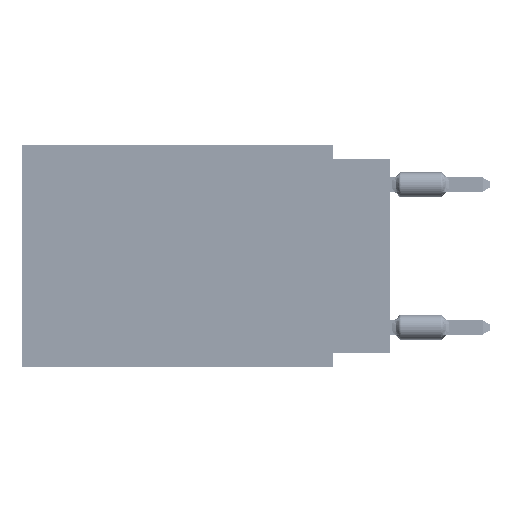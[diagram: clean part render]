
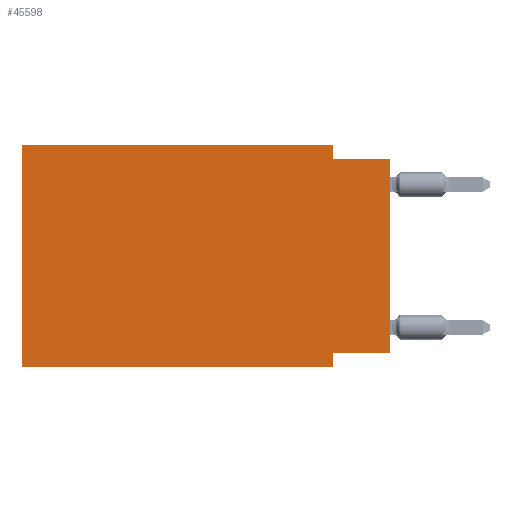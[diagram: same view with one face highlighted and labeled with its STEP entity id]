
A CAD part, left-side view. The second image highlights one B-rep face of the part: STEP entity #45598.
In plain terms, the highlighted planar face has unit normal (-1, 0, 0).
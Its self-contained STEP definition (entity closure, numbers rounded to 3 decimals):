
#2475 = DIRECTION ( 'NONE',  ( 0., -1., 0. ) ) ;
#2981 = EDGE_CURVE ( 'NONE', #34282, #34137, #37759, .T. ) ;
#3717 = VECTOR ( 'NONE', #36213, 1000. ) ;
#3864 = FACE_OUTER_BOUND ( 'NONE', #32649, .T. ) ;
#4817 = VECTOR ( 'NONE', #51112, 1000. ) ;
#5017 = DIRECTION ( 'NONE',  ( 0., -1., 0. ) ) ;
#6889 = EDGE_CURVE ( 'NONE', #23147, #39089, #38654, .T. ) ;
#7675 = VECTOR ( 'NONE', #46859, 1000. ) ;
#10499 = CARTESIAN_POINT ( 'NONE',  ( 0., 0., -0.635 ) ) ;
#12782 = CARTESIAN_POINT ( 'NONE',  ( 0., 0., -9.271 ) ) ;
#13232 = EDGE_CURVE ( 'NONE', #24584, #39089, #41303, .T. ) ;
#13261 = ORIENTED_EDGE ( 'NONE', *, *, #19563, .F. ) ;
#13818 = ORIENTED_EDGE ( 'NONE', *, *, #63103, .T. ) ;
#16431 = EDGE_CURVE ( 'NONE', #24584, #31698, #51775, .T. ) ;
#17230 = EDGE_CURVE ( 'NONE', #31698, #34282, #43219, .T. ) ;
#17714 = VECTOR ( 'NONE', #5017, 1000. ) ;
#19563 = EDGE_CURVE ( 'NONE', #34137, #33366, #47447, .T. ) ;
#22340 = CARTESIAN_POINT ( 'NONE',  ( 0., 2.54, 0. ) ) ;
#22979 = VECTOR ( 'NONE', #62501, 1000. ) ;
#23147 = VERTEX_POINT ( 'NONE', #27498 ) ;
#24584 = VERTEX_POINT ( 'NONE', #31241 ) ;
#26050 = DIRECTION ( 'NONE',  ( 0., 1., 0. ) ) ;
#27498 = CARTESIAN_POINT ( 'NONE',  ( 0., 2.54, -9.271 ) ) ;
#27573 = CARTESIAN_POINT ( 'NONE',  ( 0., 0., -0.635 ) ) ;
#27661 = VECTOR ( 'NONE', #2475, 1000. ) ;
#28936 = VECTOR ( 'NONE', #26050, 1000. ) ;
#30209 = PLANE ( 'NONE',  #43224 ) ;
#30893 = VECTOR ( 'NONE', #32599, 1000. ) ;
#31241 = CARTESIAN_POINT ( 'NONE',  ( 0., 16.383, -9.906 ) ) ;
#31698 = VERTEX_POINT ( 'NONE', #35308 ) ;
#32599 = DIRECTION ( 'NONE',  ( 0., 0., -1. ) ) ;
#32649 = EDGE_LOOP ( 'NONE', ( #13818, #13261, #65096, #48351, #55353, #58782, #36715, #64211 ) ) ;
#33366 = VERTEX_POINT ( 'NONE', #27573 ) ;
#34137 = VERTEX_POINT ( 'NONE', #36009 ) ;
#34282 = VERTEX_POINT ( 'NONE', #48649 ) ;
#35114 = VERTEX_POINT ( 'NONE', #12782 ) ;
#35246 = LINE ( 'NONE', #53352, #7675 ) ;
#35308 = CARTESIAN_POINT ( 'NONE',  ( 0., 16.383, 0. ) ) ;
#35340 = DIRECTION ( 'NONE',  ( 1., 0., 0. ) ) ;
#36009 = CARTESIAN_POINT ( 'NONE',  ( 0., 2.54, -0.635 ) ) ;
#36213 = DIRECTION ( 'NONE',  ( 0., 0., -1. ) ) ;
#36715 = ORIENTED_EDGE ( 'NONE', *, *, #6889, .F. ) ;
#37759 = LINE ( 'NONE', #22340, #30893 ) ;
#38654 = LINE ( 'NONE', #49955, #3717 ) ;
#39089 = VERTEX_POINT ( 'NONE', #59031 ) ;
#40461 = LINE ( 'NONE', #41804, #28936 ) ;
#41303 = LINE ( 'NONE', #46081, #17714 ) ;
#41804 = CARTESIAN_POINT ( 'NONE',  ( 0., 0., -9.271 ) ) ;
#43219 = LINE ( 'NONE', #60303, #27661 ) ;
#43224 = AXIS2_PLACEMENT_3D ( 'NONE', #50414, #35340, #65460 ) ;
#45598 = ADVANCED_FACE ( 'NONE', ( #3864 ), #30209, .F. ) ;
#46081 = CARTESIAN_POINT ( 'NONE',  ( 0., 16.383, -9.906 ) ) ;
#46859 = DIRECTION ( 'NONE',  ( 0., 0., 1. ) ) ;
#47447 = LINE ( 'NONE', #10499, #22979 ) ;
#48351 = ORIENTED_EDGE ( 'NONE', *, *, #17230, .F. ) ;
#48649 = CARTESIAN_POINT ( 'NONE',  ( 0., 2.54, 0. ) ) ;
#49955 = CARTESIAN_POINT ( 'NONE',  ( 0., 2.54, -9.906 ) ) ;
#50414 = CARTESIAN_POINT ( 'NONE',  ( 0., 16.383, 0. ) ) ;
#51112 = DIRECTION ( 'NONE',  ( 0., 0., 1. ) ) ;
#51775 = LINE ( 'NONE', #56899, #4817 ) ;
#53352 = CARTESIAN_POINT ( 'NONE',  ( 0., 0., 0. ) ) ;
#54534 = EDGE_CURVE ( 'NONE', #35114, #23147, #40461, .T. ) ;
#55353 = ORIENTED_EDGE ( 'NONE', *, *, #16431, .F. ) ;
#56899 = CARTESIAN_POINT ( 'NONE',  ( 0., 16.383, 0. ) ) ;
#58782 = ORIENTED_EDGE ( 'NONE', *, *, #13232, .T. ) ;
#59031 = CARTESIAN_POINT ( 'NONE',  ( 0., 2.54, -9.906 ) ) ;
#60303 = CARTESIAN_POINT ( 'NONE',  ( 0., 16.383, 0. ) ) ;
#62501 = DIRECTION ( 'NONE',  ( 0., -1., 0. ) ) ;
#63103 = EDGE_CURVE ( 'NONE', #35114, #33366, #35246, .T. ) ;
#64211 = ORIENTED_EDGE ( 'NONE', *, *, #54534, .F. ) ;
#65096 = ORIENTED_EDGE ( 'NONE', *, *, #2981, .F. ) ;
#65460 = DIRECTION ( 'NONE',  ( 0., 0., -1. ) ) ;
